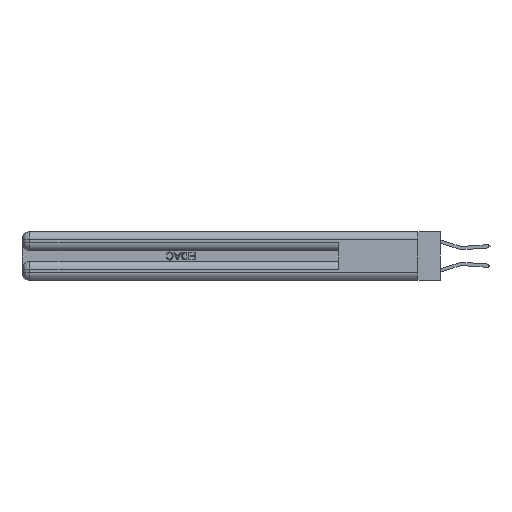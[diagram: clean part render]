
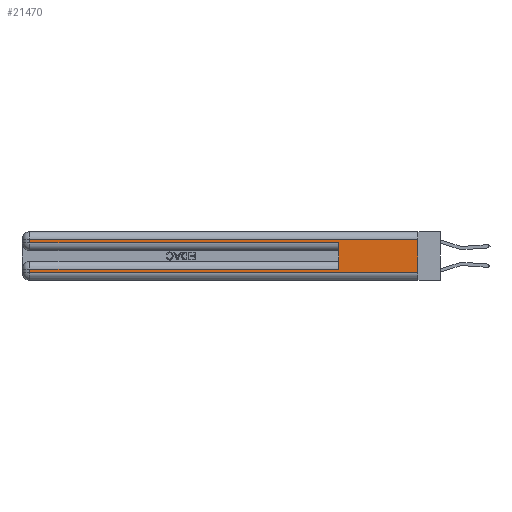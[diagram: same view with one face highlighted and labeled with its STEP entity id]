
A CAD part, left-side view. The second image highlights one B-rep face of the part: STEP entity #21470.
In plain terms, the highlighted planar face has unit normal (-1, 0, 0).
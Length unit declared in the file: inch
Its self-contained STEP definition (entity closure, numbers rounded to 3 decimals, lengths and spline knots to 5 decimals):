
#397 = VECTOR ( 'NONE', #21386, 39.37008 ) ;
#718 = VERTEX_POINT ( 'NONE', #7781 ) ;
#2784 = VERTEX_POINT ( 'NONE', #28883 ) ;
#3520 = DIRECTION ( 'NONE',  ( 0., 1., 0. ) ) ;
#4149 = VECTOR ( 'NONE', #29090, 39.37008 ) ;
#4374 = LINE ( 'NONE', #17545, #16668 ) ;
#4417 = EDGE_CURVE ( 'NONE', #2784, #8466, #6632, .T. ) ;
#4922 = EDGE_CURVE ( 'NONE', #2784, #20108, #31937, .T. ) ;
#5115 = EDGE_CURVE ( 'NONE', #27665, #11749, #26241, .T. ) ;
#5244 = DIRECTION ( 'NONE',  ( 1., 0., 0. ) ) ;
#5701 = CARTESIAN_POINT ( 'NONE',  ( 0., 0., 0.06 ) ) ;
#5806 = VECTOR ( 'NONE', #3520, 39.37008 ) ;
#6539 = LINE ( 'NONE', #5701, #397 ) ;
#6632 = LINE ( 'NONE', #21718, #5806 ) ;
#7103 = DIRECTION ( 'NONE',  ( 0., 0., -1. ) ) ;
#7515 = CARTESIAN_POINT ( 'NONE',  ( 0., 0.6, 0.285 ) ) ;
#7524 = VERTEX_POINT ( 'NONE', #25336 ) ;
#7781 = CARTESIAN_POINT ( 'NONE',  ( 0., 0., 0.06 ) ) ;
#8181 = CARTESIAN_POINT ( 'NONE',  ( 0., 0.6, 0.145 ) ) ;
#8466 = VERTEX_POINT ( 'NONE', #13715 ) ;
#8843 = FACE_OUTER_BOUND ( 'NONE', #22913, .T. ) ;
#9501 = CARTESIAN_POINT ( 'NONE',  ( 0., 0., 0.285 ) ) ;
#10576 = DIRECTION ( 'NONE',  ( 0., 0., -1. ) ) ;
#10730 = CARTESIAN_POINT ( 'NONE',  ( 0., 2.94, 0.37 ) ) ;
#11749 = VERTEX_POINT ( 'NONE', #27857 ) ;
#12155 = DIRECTION ( 'NONE',  ( 0., -1., 0. ) ) ;
#12364 = VECTOR ( 'NONE', #16786, 39.37008 ) ;
#12951 = CARTESIAN_POINT ( 'NONE',  ( 0., 0., 0.37 ) ) ;
#13715 = CARTESIAN_POINT ( 'NONE',  ( 0., 2.94, 0.085 ) ) ;
#13906 = EDGE_CURVE ( 'NONE', #11749, #7524, #31284, .T. ) ;
#14162 = CARTESIAN_POINT ( 'NONE',  ( 0., 0., 0.31 ) ) ;
#14961 = VERTEX_POINT ( 'NONE', #32714 ) ;
#16029 = DIRECTION ( 'NONE',  ( 0., 0., -1. ) ) ;
#16668 = VECTOR ( 'NONE', #7103, 39.37008 ) ;
#16786 = DIRECTION ( 'NONE',  ( 0., 1., 0. ) ) ;
#16914 = LINE ( 'NONE', #9501, #29943 ) ;
#17545 = CARTESIAN_POINT ( 'NONE',  ( 0., 0., 0.37 ) ) ;
#19315 = VECTOR ( 'NONE', #10576, 39.37008 ) ;
#19635 = ORIENTED_EDGE ( 'NONE', *, *, #31834, .T. ) ;
#20108 = VERTEX_POINT ( 'NONE', #7515 ) ;
#21386 = DIRECTION ( 'NONE',  ( 0., -1., 0. ) ) ;
#21470 = ADVANCED_FACE ( 'NONE', ( #8843 ), #28666, .F. ) ;
#21718 = CARTESIAN_POINT ( 'NONE',  ( 0., 0., 0.085 ) ) ;
#22913 = EDGE_LOOP ( 'NONE', ( #33864, #33608, #32711, #32665, #31874, #31617, #19635, #24600 ) ) ;
#23554 = DIRECTION ( 'NONE',  ( 0., 0., -1. ) ) ;
#24361 = VECTOR ( 'NONE', #16029, 39.37008 ) ;
#24600 = ORIENTED_EDGE ( 'NONE', *, *, #32488, .T. ) ;
#25336 = CARTESIAN_POINT ( 'NONE',  ( 0., 2.94, 0.285 ) ) ;
#26241 = LINE ( 'NONE', #14162, #12364 ) ;
#26248 = LINE ( 'NONE', #31341, #19315 ) ;
#27011 = CARTESIAN_POINT ( 'NONE',  ( 0., 0., 0.31 ) ) ;
#27573 = AXIS2_PLACEMENT_3D ( 'NONE', #12951, #5244, #23554 ) ;
#27665 = VERTEX_POINT ( 'NONE', #27011 ) ;
#27857 = CARTESIAN_POINT ( 'NONE',  ( 0., 2.94, 0.31 ) ) ;
#27908 = EDGE_CURVE ( 'NONE', #27665, #718, #4374, .T. ) ;
#28666 = PLANE ( 'NONE',  #27573 ) ;
#28883 = CARTESIAN_POINT ( 'NONE',  ( 0., 0.6, 0.085 ) ) ;
#29090 = DIRECTION ( 'NONE',  ( 0., 0., 1. ) ) ;
#29943 = VECTOR ( 'NONE', #12155, 39.37008 ) ;
#30951 = EDGE_CURVE ( 'NONE', #7524, #20108, #16914, .T. ) ;
#31284 = LINE ( 'NONE', #10730, #24361 ) ;
#31341 = CARTESIAN_POINT ( 'NONE',  ( 0., 2.94, 0.37 ) ) ;
#31617 = ORIENTED_EDGE ( 'NONE', *, *, #4417, .T. ) ;
#31834 = EDGE_CURVE ( 'NONE', #8466, #14961, #26248, .T. ) ;
#31874 = ORIENTED_EDGE ( 'NONE', *, *, #4922, .F. ) ;
#31937 = LINE ( 'NONE', #8181, #4149 ) ;
#32488 = EDGE_CURVE ( 'NONE', #14961, #718, #6539, .T. ) ;
#32665 = ORIENTED_EDGE ( 'NONE', *, *, #30951, .T. ) ;
#32711 = ORIENTED_EDGE ( 'NONE', *, *, #13906, .T. ) ;
#32714 = CARTESIAN_POINT ( 'NONE',  ( 0., 2.94, 0.06 ) ) ;
#33608 = ORIENTED_EDGE ( 'NONE', *, *, #5115, .T. ) ;
#33864 = ORIENTED_EDGE ( 'NONE', *, *, #27908, .F. ) ;
